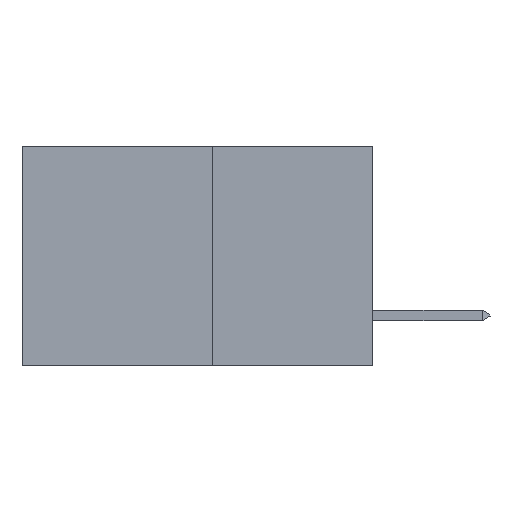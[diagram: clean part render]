
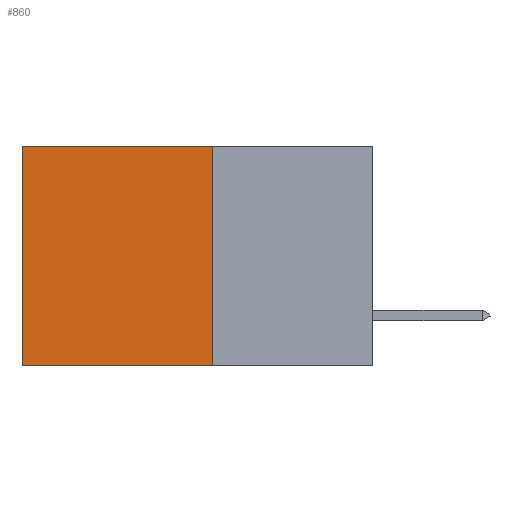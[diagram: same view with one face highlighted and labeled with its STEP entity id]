
A CAD part, left-side view. The second image highlights one B-rep face of the part: STEP entity #860.
In plain terms, the highlighted planar face has unit normal (-1, 0, 0).
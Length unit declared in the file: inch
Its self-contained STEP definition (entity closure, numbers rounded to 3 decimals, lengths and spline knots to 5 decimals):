
#304 = CARTESIAN_POINT ( 'NONE',  ( 0.277, 0.59, 0. ) ) ;
#426 = VERTEX_POINT ( 'NONE', #12214 ) ;
#830 = ORIENTED_EDGE ( 'NONE', *, *, #1476, .T. ) ;
#860 = ADVANCED_FACE ( 'NONE', ( #5770 ), #8835, .F. ) ;
#1476 = EDGE_CURVE ( 'NONE', #8595, #2399, #6577, .T. ) ;
#1666 = CARTESIAN_POINT ( 'NONE',  ( 0.277, 0.27, 0. ) ) ;
#2119 = VERTEX_POINT ( 'NONE', #4542 ) ;
#2256 = LINE ( 'NONE', #6305, #8005 ) ;
#2399 = VERTEX_POINT ( 'NONE', #304 ) ;
#2948 = EDGE_LOOP ( 'NONE', ( #9553, #10828, #7752, #830 ) ) ;
#2971 = VECTOR ( 'NONE', #3168, 39.37008 ) ;
#3168 = DIRECTION ( 'NONE',  ( 0., 1., 0. ) ) ;
#3196 = CARTESIAN_POINT ( 'NONE',  ( 0.277, 0.27, -0.37 ) ) ;
#3631 = EDGE_CURVE ( 'NONE', #2399, #2119, #9814, .T. ) ;
#4542 = CARTESIAN_POINT ( 'NONE',  ( 0.277, 0.59, -0.37 ) ) ;
#5377 = DIRECTION ( 'NONE',  ( 1., 0., 0. ) ) ;
#5564 = DIRECTION ( 'NONE',  ( 0., 1., 0. ) ) ;
#5770 = FACE_OUTER_BOUND ( 'NONE', #2948, .T. ) ;
#6305 = CARTESIAN_POINT ( 'NONE',  ( 0.277, 0.27, -0.37 ) ) ;
#6577 = LINE ( 'NONE', #7078, #8780 ) ;
#7078 = CARTESIAN_POINT ( 'NONE',  ( 0.277, 0.27, 0. ) ) ;
#7752 = ORIENTED_EDGE ( 'NONE', *, *, #11406, .F. ) ;
#7993 = DIRECTION ( 'NONE',  ( 0., 0., -1. ) ) ;
#8005 = VECTOR ( 'NONE', #12170, 39.37008 ) ;
#8081 = LINE ( 'NONE', #3196, #2971 ) ;
#8168 = EDGE_CURVE ( 'NONE', #426, #2119, #8081, .T. ) ;
#8595 = VERTEX_POINT ( 'NONE', #1666 ) ;
#8780 = VECTOR ( 'NONE', #5564, 39.37008 ) ;
#8835 = PLANE ( 'NONE',  #8838 ) ;
#8838 = AXIS2_PLACEMENT_3D ( 'NONE', #9115, #5377, #11503 ) ;
#9115 = CARTESIAN_POINT ( 'NONE',  ( 0.277, 0.27, -0.37 ) ) ;
#9553 = ORIENTED_EDGE ( 'NONE', *, *, #3631, .T. ) ;
#9814 = LINE ( 'NONE', #11076, #10130 ) ;
#10130 = VECTOR ( 'NONE', #7993, 39.37008 ) ;
#10828 = ORIENTED_EDGE ( 'NONE', *, *, #8168, .F. ) ;
#11076 = CARTESIAN_POINT ( 'NONE',  ( 0.277, 0.59, -0.37 ) ) ;
#11406 = EDGE_CURVE ( 'NONE', #8595, #426, #2256, .T. ) ;
#11503 = DIRECTION ( 'NONE',  ( 0., 0., -1. ) ) ;
#12170 = DIRECTION ( 'NONE',  ( 0., 0., -1. ) ) ;
#12214 = CARTESIAN_POINT ( 'NONE',  ( 0.277, 0.27, -0.37 ) ) ;
